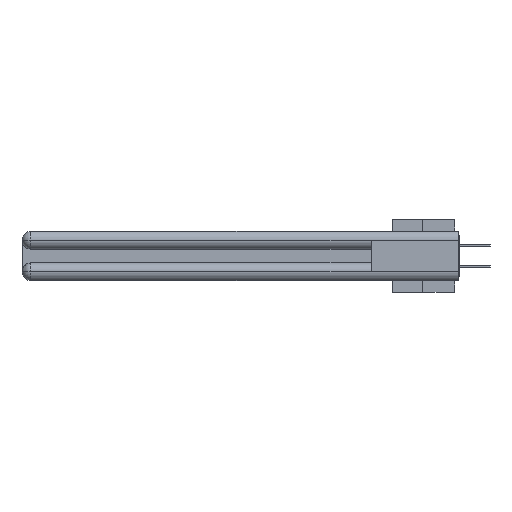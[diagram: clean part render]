
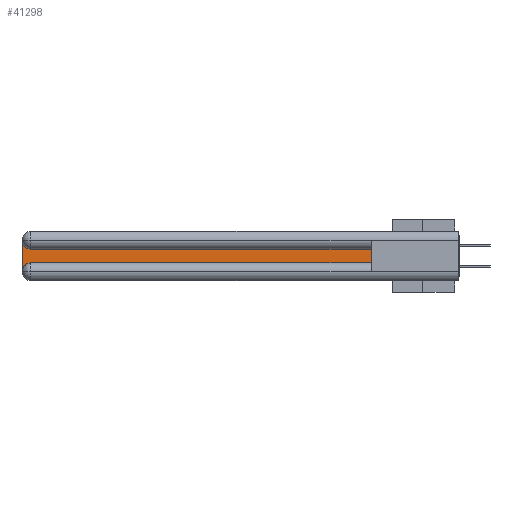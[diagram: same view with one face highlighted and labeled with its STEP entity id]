
A CAD part, left-side view. The second image highlights one B-rep face of the part: STEP entity #41298.
In plain terms, the highlighted planar face has unit normal (-1, 0, 0).
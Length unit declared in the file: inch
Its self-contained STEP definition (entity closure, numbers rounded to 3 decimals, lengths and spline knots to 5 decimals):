
#35 = VERTEX_POINT ( 'NONE', #8834 ) ;
#1004 = DIRECTION ( 'NONE',  ( 0., -1., 0. ) ) ;
#1423 = VERTEX_POINT ( 'NONE', #2765 ) ;
#1583 = CARTESIAN_POINT ( 'NONE',  ( 0.075, 3., -0.1225 ) ) ;
#1765 = CARTESIAN_POINT ( 'NONE',  ( 0.075, 2.94, -0.0625 ) ) ;
#1798 = VECTOR ( 'NONE', #1004, 39.37008 ) ;
#2334 = CARTESIAN_POINT ( 'NONE',  ( 0.075, 2.94, -0.2175 ) ) ;
#2765 = CARTESIAN_POINT ( 'NONE',  ( 0.075, 0.6, -0.1225 ) ) ;
#5636 = CARTESIAN_POINT ( 'NONE',  ( 0.075, 3., -0.2175 ) ) ;
#6205 = VERTEX_POINT ( 'NONE', #2334 ) ;
#6250 = ORIENTED_EDGE ( 'NONE', *, *, #30627, .T. ) ;
#7155 = DIRECTION ( 'NONE',  ( 0., 0., 1. ) ) ;
#8632 = DIRECTION ( 'NONE',  ( 1., 0., 0. ) ) ;
#8834 = CARTESIAN_POINT ( 'NONE',  ( 0.075, 3., -0.2775 ) ) ;
#9229 = EDGE_CURVE ( 'NONE', #1423, #14776, #36651, .T. ) ;
#9429 = LINE ( 'NONE', #25058, #1798 ) ;
#9781 = FACE_OUTER_BOUND ( 'NONE', #39882, .T. ) ;
#10993 = EDGE_CURVE ( 'NONE', #33230, #1423, #37905, .T. ) ;
#11786 = CARTESIAN_POINT ( 'NONE',  ( 0.075, 2.94, -0.2775 ) ) ;
#12860 = DIRECTION ( 'NONE',  ( 1., 0., 0. ) ) ;
#13130 = EDGE_CURVE ( 'NONE', #6205, #33230, #9429, .T. ) ;
#14673 = CARTESIAN_POINT ( 'NONE',  ( 0.075, 0.6, -0.1225 ) ) ;
#14776 = VERTEX_POINT ( 'NONE', #20156 ) ;
#16465 = VECTOR ( 'NONE', #42513, 39.37008 ) ;
#16878 = CARTESIAN_POINT ( 'NONE',  ( 0.075, 0.6, -0.2175 ) ) ;
#17448 = CARTESIAN_POINT ( 'NONE',  ( 0.075, 0.6, -0.2175 ) ) ;
#18929 = DIRECTION ( 'NONE',  ( 1., 0., 0. ) ) ;
#18942 = PLANE ( 'NONE',  #24791 ) ;
#20156 = CARTESIAN_POINT ( 'NONE',  ( 0.075, 2.94, -0.1225 ) ) ;
#20617 = CIRCLE ( 'NONE', #30068, 0.06 ) ;
#21246 = AXIS2_PLACEMENT_3D ( 'NONE', #11786, #18929, #43272 ) ;
#22362 = ORIENTED_EDGE ( 'NONE', *, *, #40723, .T. ) ;
#22778 = CARTESIAN_POINT ( 'NONE',  ( 0.075, 3., -0.0625 ) ) ;
#24791 = AXIS2_PLACEMENT_3D ( 'NONE', #1583, #12860, #30328 ) ;
#25058 = CARTESIAN_POINT ( 'NONE',  ( 0.075, 0.6, -0.2175 ) ) ;
#25607 = CIRCLE ( 'NONE', #21246, 0.06 ) ;
#25873 = LINE ( 'NONE', #5636, #29135 ) ;
#26952 = EDGE_CURVE ( 'NONE', #36972, #35, #25873, .T. ) ;
#29135 = VECTOR ( 'NONE', #33313, 39.37008 ) ;
#30068 = AXIS2_PLACEMENT_3D ( 'NONE', #1765, #8632, #36306 ) ;
#30328 = DIRECTION ( 'NONE',  ( 0., 0., -1. ) ) ;
#30627 = EDGE_CURVE ( 'NONE', #14776, #36972, #20617, .T. ) ;
#33230 = VERTEX_POINT ( 'NONE', #16878 ) ;
#33313 = DIRECTION ( 'NONE',  ( 0., 0., -1. ) ) ;
#33574 = ORIENTED_EDGE ( 'NONE', *, *, #26952, .T. ) ;
#34267 = ORIENTED_EDGE ( 'NONE', *, *, #9229, .T. ) ;
#35187 = ORIENTED_EDGE ( 'NONE', *, *, #13130, .T. ) ;
#36306 = DIRECTION ( 'NONE',  ( 0., 0., -1. ) ) ;
#36651 = LINE ( 'NONE', #14673, #16465 ) ;
#36972 = VERTEX_POINT ( 'NONE', #22778 ) ;
#37905 = LINE ( 'NONE', #17448, #44467 ) ;
#39882 = EDGE_LOOP ( 'NONE', ( #34267, #6250, #33574, #22362, #35187, #42347 ) ) ;
#40723 = EDGE_CURVE ( 'NONE', #35, #6205, #25607, .T. ) ;
#41298 = ADVANCED_FACE ( 'NONE', ( #9781 ), #18942, .F. ) ;
#42347 = ORIENTED_EDGE ( 'NONE', *, *, #10993, .T. ) ;
#42513 = DIRECTION ( 'NONE',  ( 0., 1., 0. ) ) ;
#43272 = DIRECTION ( 'NONE',  ( 0., 0., -1. ) ) ;
#44467 = VECTOR ( 'NONE', #7155, 39.37008 ) ;
